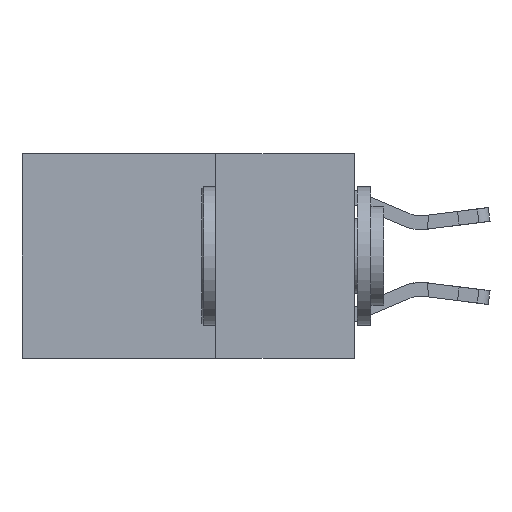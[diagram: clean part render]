
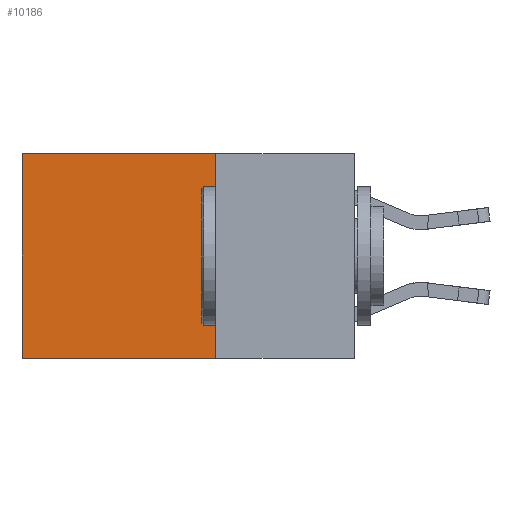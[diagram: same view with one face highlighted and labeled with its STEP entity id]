
A CAD part, left-side view. The second image highlights one B-rep face of the part: STEP entity #10186.
In plain terms, the highlighted planar face has unit normal (-1, 0, 0).
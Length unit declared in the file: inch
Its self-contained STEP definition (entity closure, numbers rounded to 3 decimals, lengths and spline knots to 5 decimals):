
#180 = CARTESIAN_POINT ( 'NONE',  ( 0.2625, 0.6, 0. ) ) ;
#961 = VERTEX_POINT ( 'NONE', #4771 ) ;
#1151 = CARTESIAN_POINT ( 'NONE',  ( 0.2625, 0.25, -0.37 ) ) ;
#1348 = DIRECTION ( 'NONE',  ( 0., 1., 0. ) ) ;
#1648 = CARTESIAN_POINT ( 'NONE',  ( 0.2625, 0.25, 0. ) ) ;
#1812 = CARTESIAN_POINT ( 'NONE',  ( 0.2625, 0.25, 0. ) ) ;
#2220 = VECTOR ( 'NONE', #5776, 39.37008 ) ;
#3340 = VERTEX_POINT ( 'NONE', #180 ) ;
#3561 = ORIENTED_EDGE ( 'NONE', *, *, #16593, .T. ) ;
#4771 = CARTESIAN_POINT ( 'NONE',  ( 0.2625, 0.6, -0.37 ) ) ;
#5335 = FACE_OUTER_BOUND ( 'NONE', #14599, .T. ) ;
#5692 = VECTOR ( 'NONE', #9477, 39.37008 ) ;
#5776 = DIRECTION ( 'NONE',  ( 0., 1., 0. ) ) ;
#6021 = EDGE_CURVE ( 'NONE', #17959, #11606, #18880, .T. ) ;
#7063 = PLANE ( 'NONE',  #7185 ) ;
#7104 = VECTOR ( 'NONE', #11625, 39.37008 ) ;
#7185 = AXIS2_PLACEMENT_3D ( 'NONE', #17713, #16180, #18007 ) ;
#7778 = CARTESIAN_POINT ( 'NONE',  ( 0.2625, 0.25, -0.37 ) ) ;
#9412 = VECTOR ( 'NONE', #1348, 39.37008 ) ;
#9477 = DIRECTION ( 'NONE',  ( 0., 0., -1. ) ) ;
#10186 = ADVANCED_FACE ( 'NONE', ( #5335 ), #7063, .F. ) ;
#10431 = LINE ( 'NONE', #19673, #2220 ) ;
#10635 = ORIENTED_EDGE ( 'NONE', *, *, #6021, .F. ) ;
#11606 = VERTEX_POINT ( 'NONE', #7778 ) ;
#11625 = DIRECTION ( 'NONE',  ( 0., 0., -1. ) ) ;
#13307 = LINE ( 'NONE', #19510, #7104 ) ;
#14127 = ORIENTED_EDGE ( 'NONE', *, *, #14287, .T. ) ;
#14287 = EDGE_CURVE ( 'NONE', #3340, #961, #13307, .T. ) ;
#14408 = EDGE_CURVE ( 'NONE', #11606, #961, #15345, .T. ) ;
#14599 = EDGE_LOOP ( 'NONE', ( #14127, #18094, #10635, #3561 ) ) ;
#15345 = LINE ( 'NONE', #1151, #9412 ) ;
#16180 = DIRECTION ( 'NONE',  ( 1., 0., 0. ) ) ;
#16593 = EDGE_CURVE ( 'NONE', #17959, #3340, #10431, .T. ) ;
#17713 = CARTESIAN_POINT ( 'NONE',  ( 0.2625, 0.25, 0. ) ) ;
#17959 = VERTEX_POINT ( 'NONE', #1812 ) ;
#18007 = DIRECTION ( 'NONE',  ( 0., 0., -1. ) ) ;
#18094 = ORIENTED_EDGE ( 'NONE', *, *, #14408, .F. ) ;
#18880 = LINE ( 'NONE', #1648, #5692 ) ;
#19510 = CARTESIAN_POINT ( 'NONE',  ( 0.2625, 0.6, 0. ) ) ;
#19673 = CARTESIAN_POINT ( 'NONE',  ( 0.2625, 0.25, 0. ) ) ;
